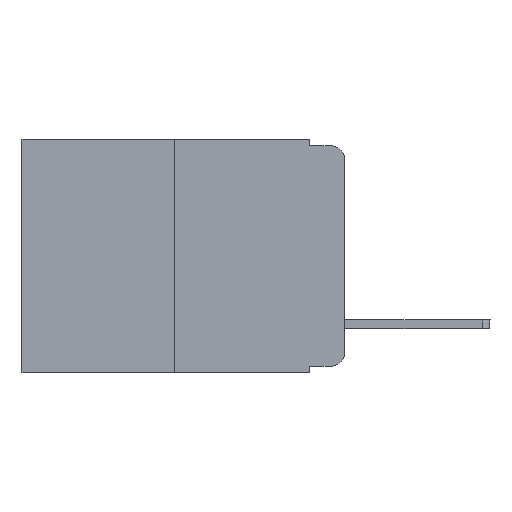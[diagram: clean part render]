
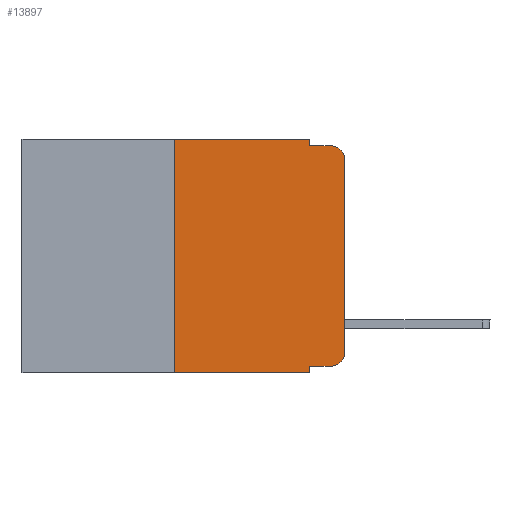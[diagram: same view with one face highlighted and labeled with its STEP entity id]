
A CAD part, left-side view. The second image highlights one B-rep face of the part: STEP entity #13897.
In plain terms, the highlighted planar face has unit normal (-1, 0, 0).
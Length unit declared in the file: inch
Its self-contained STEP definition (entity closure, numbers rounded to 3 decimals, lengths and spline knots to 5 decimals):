
#632 = CARTESIAN_POINT ( 'NONE',  ( 0., 0.051, -0.343 ) ) ;
#694 = EDGE_CURVE ( 'NONE', #9114, #7357, #8259, .T. ) ;
#774 = ORIENTED_EDGE ( 'NONE', *, *, #7031, .T. ) ;
#999 = ORIENTED_EDGE ( 'NONE', *, *, #8202, .F. ) ;
#1308 = CARTESIAN_POINT ( 'NONE',  ( 0., 0.02, -0.03 ) ) ;
#1620 = DIRECTION ( 'NONE',  ( 0., -1., 0. ) ) ;
#1801 = VECTOR ( 'NONE', #5804, 39.37008 ) ;
#2122 = EDGE_CURVE ( 'NONE', #7357, #16971, #5338, .T. ) ;
#2227 = VECTOR ( 'NONE', #10736, 39.37008 ) ;
#2404 = CIRCLE ( 'NONE', #5027, 0.02 ) ;
#2715 = VERTEX_POINT ( 'NONE', #22058 ) ;
#2866 = FACE_OUTER_BOUND ( 'NONE', #6595, .T. ) ;
#2956 = ORIENTED_EDGE ( 'NONE', *, *, #694, .T. ) ;
#3060 = DIRECTION ( 'NONE',  ( 0., 0., -1. ) ) ;
#3097 = EDGE_CURVE ( 'NONE', #19754, #7143, #15934, .T. ) ;
#3225 = VERTEX_POINT ( 'NONE', #632 ) ;
#3388 = ORIENTED_EDGE ( 'NONE', *, *, #11681, .F. ) ;
#3482 = LINE ( 'NONE', #12778, #8513 ) ;
#3633 = CARTESIAN_POINT ( 'NONE',  ( 0., 0.473, 0. ) ) ;
#3970 = DIRECTION ( 'NONE',  ( 0., 0., -1. ) ) ;
#4044 = CARTESIAN_POINT ( 'NONE',  ( 0., 0.25, 0. ) ) ;
#4255 = DIRECTION ( 'NONE',  ( 0., 0., 1. ) ) ;
#4486 = CARTESIAN_POINT ( 'NONE',  ( 0., 0.25, 0. ) ) ;
#4851 = CARTESIAN_POINT ( 'NONE',  ( 0., 0.051, -0.333 ) ) ;
#5027 = AXIS2_PLACEMENT_3D ( 'NONE', #22917, #12357, #15641 ) ;
#5338 = CIRCLE ( 'NONE', #22577, 0.02 ) ;
#5700 = ORIENTED_EDGE ( 'NONE', *, *, #17611, .F. ) ;
#5804 = DIRECTION ( 'NONE',  ( 0., -1., 0. ) ) ;
#5834 = CARTESIAN_POINT ( 'NONE',  ( 0., 0.051, 0. ) ) ;
#6222 = DIRECTION ( 'NONE',  ( 0., -1., 0. ) ) ;
#6595 = EDGE_LOOP ( 'NONE', ( #2956, #19240, #3388, #999, #9750, #14034, #20019, #5700, #19474, #774 ) ) ;
#6613 = DIRECTION ( 'NONE',  ( -1., 0., 0. ) ) ;
#6850 = VECTOR ( 'NONE', #1620, 39.37008 ) ;
#7031 = EDGE_CURVE ( 'NONE', #7143, #9114, #2404, .T. ) ;
#7142 = DIRECTION ( 'NONE',  ( 0., -1., 0. ) ) ;
#7143 = VERTEX_POINT ( 'NONE', #17743 ) ;
#7357 = VERTEX_POINT ( 'NONE', #12214 ) ;
#8146 = VECTOR ( 'NONE', #3970, 39.37008 ) ;
#8202 = EDGE_CURVE ( 'NONE', #18696, #2715, #21916, .T. ) ;
#8259 = LINE ( 'NONE', #15410, #15052 ) ;
#8369 = DIRECTION ( 'NONE',  ( 0., 0., 1. ) ) ;
#8428 = VECTOR ( 'NONE', #4255, 39.37008 ) ;
#8513 = VECTOR ( 'NONE', #7142, 39.37008 ) ;
#9114 = VERTEX_POINT ( 'NONE', #13839 ) ;
#9390 = CARTESIAN_POINT ( 'NONE',  ( 0., 0.051, 0. ) ) ;
#9750 = ORIENTED_EDGE ( 'NONE', *, *, #9934, .F. ) ;
#9934 = EDGE_CURVE ( 'NONE', #19739, #18696, #17734, .T. ) ;
#10063 = CARTESIAN_POINT ( 'NONE',  ( 0., 0.473, 0. ) ) ;
#10541 = VERTEX_POINT ( 'NONE', #20043 ) ;
#10681 = LINE ( 'NONE', #22993, #6850 ) ;
#10736 = DIRECTION ( 'NONE',  ( 0., 0., -1. ) ) ;
#11594 = DIRECTION ( 'NONE',  ( 1., 0., 0. ) ) ;
#11681 = EDGE_CURVE ( 'NONE', #2715, #16971, #10681, .T. ) ;
#11768 = LINE ( 'NONE', #4486, #8428 ) ;
#12214 = CARTESIAN_POINT ( 'NONE',  ( 0., 0., -0.03 ) ) ;
#12357 = DIRECTION ( 'NONE',  ( -1., 0., 0. ) ) ;
#12457 = CARTESIAN_POINT ( 'NONE',  ( 0., 0.02, -0.01 ) ) ;
#12778 = CARTESIAN_POINT ( 'NONE',  ( 0., 0.473, -0.343 ) ) ;
#13345 = EDGE_CURVE ( 'NONE', #10541, #19739, #11768, .T. ) ;
#13839 = CARTESIAN_POINT ( 'NONE',  ( 0., 0., -0.313 ) ) ;
#13897 = ADVANCED_FACE ( 'NONE', ( #2866 ), #20510, .F. ) ;
#14034 = ORIENTED_EDGE ( 'NONE', *, *, #13345, .F. ) ;
#14058 = AXIS2_PLACEMENT_3D ( 'NONE', #10063, #11594, #20849 ) ;
#14282 = VECTOR ( 'NONE', #6222, 39.37008 ) ;
#15052 = VECTOR ( 'NONE', #8369, 39.37008 ) ;
#15410 = CARTESIAN_POINT ( 'NONE',  ( 0., 0., 0. ) ) ;
#15641 = DIRECTION ( 'NONE',  ( 0., 0., -1. ) ) ;
#15934 = LINE ( 'NONE', #17463, #1801 ) ;
#16971 = VERTEX_POINT ( 'NONE', #12457 ) ;
#16999 = LINE ( 'NONE', #18414, #8146 ) ;
#17461 = EDGE_CURVE ( 'NONE', #10541, #3225, #3482, .T. ) ;
#17463 = CARTESIAN_POINT ( 'NONE',  ( 0., 0.051, -0.333 ) ) ;
#17611 = EDGE_CURVE ( 'NONE', #19754, #3225, #16999, .T. ) ;
#17734 = LINE ( 'NONE', #3633, #14282 ) ;
#17743 = CARTESIAN_POINT ( 'NONE',  ( 0., 0.02, -0.333 ) ) ;
#18414 = CARTESIAN_POINT ( 'NONE',  ( 0., 0.051, 0. ) ) ;
#18696 = VERTEX_POINT ( 'NONE', #9390 ) ;
#19240 = ORIENTED_EDGE ( 'NONE', *, *, #2122, .T. ) ;
#19474 = ORIENTED_EDGE ( 'NONE', *, *, #3097, .T. ) ;
#19739 = VERTEX_POINT ( 'NONE', #4044 ) ;
#19754 = VERTEX_POINT ( 'NONE', #4851 ) ;
#20019 = ORIENTED_EDGE ( 'NONE', *, *, #17461, .T. ) ;
#20043 = CARTESIAN_POINT ( 'NONE',  ( 0., 0.25, -0.343 ) ) ;
#20510 = PLANE ( 'NONE',  #14058 ) ;
#20849 = DIRECTION ( 'NONE',  ( 0., 0., -1. ) ) ;
#21916 = LINE ( 'NONE', #5834, #2227 ) ;
#22058 = CARTESIAN_POINT ( 'NONE',  ( 0., 0.051, -0.01 ) ) ;
#22577 = AXIS2_PLACEMENT_3D ( 'NONE', #1308, #6613, #3060 ) ;
#22917 = CARTESIAN_POINT ( 'NONE',  ( 0., 0.02, -0.313 ) ) ;
#22993 = CARTESIAN_POINT ( 'NONE',  ( 0., 0.051, -0.01 ) ) ;
